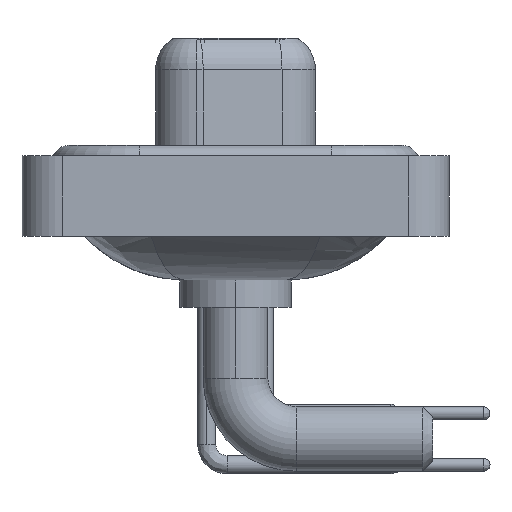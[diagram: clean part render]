
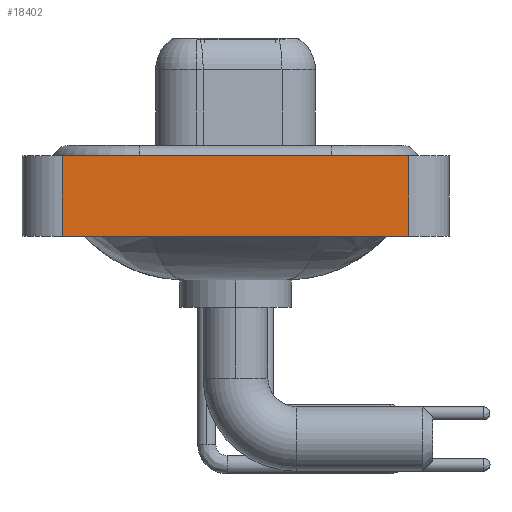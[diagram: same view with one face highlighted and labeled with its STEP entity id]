
A CAD part, left-side view. The second image highlights one B-rep face of the part: STEP entity #18402.
In plain terms, the highlighted planar face has unit normal (-1, 0, 0).
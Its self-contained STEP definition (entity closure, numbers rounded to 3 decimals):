
#1140 = EDGE_CURVE ( 'NONE', #8766, #6691, #3694, .T. ) ;
#2824 = EDGE_LOOP ( 'NONE', ( #5419, #14676, #6321, #18210 ) ) ;
#2839 = DIRECTION ( 'NONE',  ( 0., 0., 1. ) ) ;
#3565 = AXIS2_PLACEMENT_3D ( 'NONE', #10693, #4224, #12500 ) ;
#3694 = LINE ( 'NONE', #15149, #10410 ) ;
#4224 = DIRECTION ( 'NONE',  ( -1., 0., 0. ) ) ;
#4800 = LINE ( 'NONE', #6189, #19438 ) ;
#5419 = ORIENTED_EDGE ( 'NONE', *, *, #19353, .T. ) ;
#5666 = CARTESIAN_POINT ( 'NONE',  ( -7.35, 8.55, 0.4 ) ) ;
#5841 = EDGE_CURVE ( 'NONE', #13529, #10013, #4800, .T. ) ;
#5995 = DIRECTION ( 'NONE',  ( 0., -1., 0. ) ) ;
#6189 = CARTESIAN_POINT ( 'NONE',  ( -7.35, -8.55, -3.6 ) ) ;
#6321 = ORIENTED_EDGE ( 'NONE', *, *, #7073, .F. ) ;
#6691 = VERTEX_POINT ( 'NONE', #16428 ) ;
#7073 = EDGE_CURVE ( 'NONE', #13529, #8766, #17775, .T. ) ;
#8766 = VERTEX_POINT ( 'NONE', #5666 ) ;
#10013 = VERTEX_POINT ( 'NONE', #16301 ) ;
#10410 = VECTOR ( 'NONE', #16840, 1000. ) ;
#10693 = CARTESIAN_POINT ( 'NONE',  ( -7.35, -8.55, -3.6 ) ) ;
#12500 = DIRECTION ( 'NONE',  ( 0., 0., 1. ) ) ;
#12786 = CARTESIAN_POINT ( 'NONE',  ( -7.35, -8.55, -3.6 ) ) ;
#13529 = VERTEX_POINT ( 'NONE', #17232 ) ;
#13956 = LINE ( 'NONE', #12786, #16966 ) ;
#14676 = ORIENTED_EDGE ( 'NONE', *, *, #1140, .F. ) ;
#15149 = CARTESIAN_POINT ( 'NONE',  ( -7.35, -8.55, 0.4 ) ) ;
#15970 = CARTESIAN_POINT ( 'NONE',  ( -7.35, 8.55, -3.6 ) ) ;
#16301 = CARTESIAN_POINT ( 'NONE',  ( -7.35, -8.55, -3.6 ) ) ;
#16428 = CARTESIAN_POINT ( 'NONE',  ( -7.35, -8.55, 0.4 ) ) ;
#16840 = DIRECTION ( 'NONE',  ( 0., -1., 0. ) ) ;
#16966 = VECTOR ( 'NONE', #2839, 1000. ) ;
#17232 = CARTESIAN_POINT ( 'NONE',  ( -7.35, 8.55, -3.6 ) ) ;
#17265 = FACE_OUTER_BOUND ( 'NONE', #2824, .T. ) ;
#17775 = LINE ( 'NONE', #15970, #19506 ) ;
#18210 = ORIENTED_EDGE ( 'NONE', *, *, #5841, .T. ) ;
#18402 = ADVANCED_FACE ( 'NONE', ( #17265 ), #18868, .T. ) ;
#18868 = PLANE ( 'NONE',  #3565 ) ;
#19351 = DIRECTION ( 'NONE',  ( 0., 0., 1. ) ) ;
#19353 = EDGE_CURVE ( 'NONE', #10013, #6691, #13956, .T. ) ;
#19438 = VECTOR ( 'NONE', #5995, 1000. ) ;
#19506 = VECTOR ( 'NONE', #19351, 1000. ) ;
